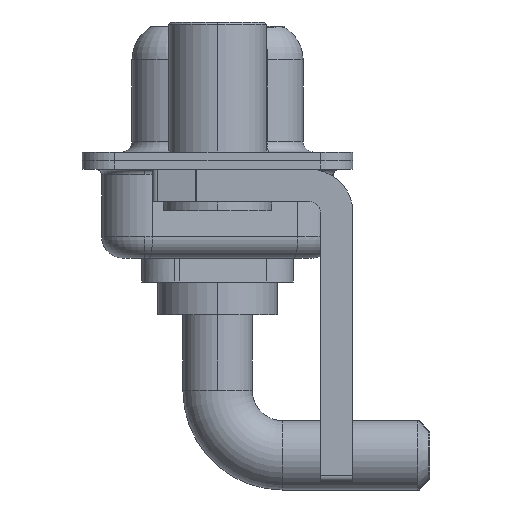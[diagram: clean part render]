
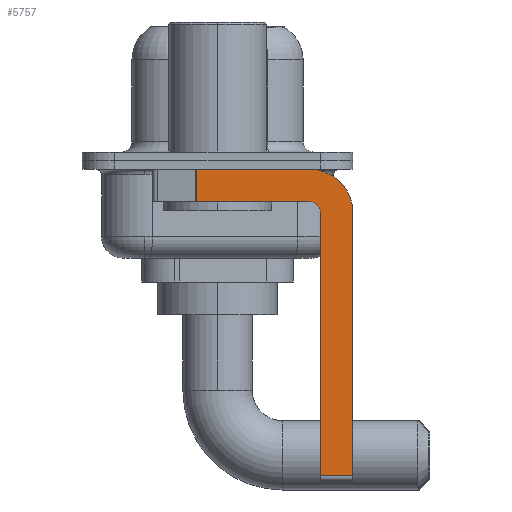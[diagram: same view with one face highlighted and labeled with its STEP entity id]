
A CAD part, left-side view. The second image highlights one B-rep face of the part: STEP entity #5757.
In plain terms, the highlighted planar face has unit normal (-1, 0, 0).
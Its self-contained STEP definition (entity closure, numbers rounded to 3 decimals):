
#242 = EDGE_CURVE ( 'NONE', #12646, #14776, #2877, .T. ) ;
#932 = CARTESIAN_POINT ( 'NONE',  ( -2.9, -6.25, -2.4 ) ) ;
#2519 = CARTESIAN_POINT ( 'NONE',  ( -2.9, -4.25, -1.9 ) ) ;
#2877 = LINE ( 'NONE', #10186, #12741 ) ;
#2991 = CIRCLE ( 'NONE', #9541, 2. ) ;
#3051 = VERTEX_POINT ( 'NONE', #7050 ) ;
#3181 = EDGE_LOOP ( 'NONE', ( #15367, #10333, #6201, #6462, #7003, #6808, #8947, #4265 ) ) ;
#3456 = CARTESIAN_POINT ( 'NONE',  ( -2.9, 0.978, -1.9 ) ) ;
#3582 = VERTEX_POINT ( 'NONE', #932 ) ;
#3919 = EDGE_CURVE ( 'NONE', #12646, #3051, #14127, .T. ) ;
#4265 = ORIENTED_EDGE ( 'NONE', *, *, #7021, .F. ) ;
#4307 = CARTESIAN_POINT ( 'NONE',  ( -2.9, -4.25, -14.55 ) ) ;
#4573 = VERTEX_POINT ( 'NONE', #7297 ) ;
#5104 = FACE_OUTER_BOUND ( 'NONE', #3181, .T. ) ;
#5132 = DIRECTION ( 'NONE',  ( 0., 0., -1. ) ) ;
#5217 = LINE ( 'NONE', #11481, #15758 ) ;
#5271 = LINE ( 'NONE', #9194, #6204 ) ;
#5757 = ADVANCED_FACE ( 'NONE', ( #5104 ), #8957, .F. ) ;
#5773 = AXIS2_PLACEMENT_3D ( 'NONE', #9042, #13033, #10471 ) ;
#6201 = ORIENTED_EDGE ( 'NONE', *, *, #6838, .F. ) ;
#6204 = VECTOR ( 'NONE', #9020, 1000. ) ;
#6462 = ORIENTED_EDGE ( 'NONE', *, *, #15039, .F. ) ;
#6474 = LINE ( 'NONE', #2519, #10650 ) ;
#6613 = DIRECTION ( 'NONE',  ( 0., -1., 0. ) ) ;
#6808 = ORIENTED_EDGE ( 'NONE', *, *, #3919, .T. ) ;
#6838 = EDGE_CURVE ( 'NONE', #8232, #13941, #6474, .T. ) ;
#7003 = ORIENTED_EDGE ( 'NONE', *, *, #242, .F. ) ;
#7021 = EDGE_CURVE ( 'NONE', #4573, #3582, #2991, .T. ) ;
#7050 = CARTESIAN_POINT ( 'NONE',  ( -2.9, -6.25, -14.55 ) ) ;
#7297 = CARTESIAN_POINT ( 'NONE',  ( -2.9, -4.25, -0.4 ) ) ;
#8232 = VERTEX_POINT ( 'NONE', #13463 ) ;
#8871 = EDGE_CURVE ( 'NONE', #13799, #13941, #13757, .T. ) ;
#8899 = CIRCLE ( 'NONE', #5773, 0.5 ) ;
#8947 = ORIENTED_EDGE ( 'NONE', *, *, #11909, .F. ) ;
#8957 = PLANE ( 'NONE',  #11171 ) ;
#9020 = DIRECTION ( 'NONE',  ( 0., -1., 0. ) ) ;
#9042 = CARTESIAN_POINT ( 'NONE',  ( -2.9, -4.25, -2.4 ) ) ;
#9194 = CARTESIAN_POINT ( 'NONE',  ( -2.9, 3., -0.4 ) ) ;
#9541 = AXIS2_PLACEMENT_3D ( 'NONE', #15632, #13074, #14486 ) ;
#10186 = CARTESIAN_POINT ( 'NONE',  ( -2.9, -4.75, -14.8 ) ) ;
#10281 = EDGE_CURVE ( 'NONE', #13799, #4573, #5271, .T. ) ;
#10333 = ORIENTED_EDGE ( 'NONE', *, *, #8871, .T. ) ;
#10471 = DIRECTION ( 'NONE',  ( 0., 0., 1. ) ) ;
#10650 = VECTOR ( 'NONE', #13903, 1000. ) ;
#10805 = CARTESIAN_POINT ( 'NONE',  ( -2.9, -4.75, -14.55 ) ) ;
#10818 = CARTESIAN_POINT ( 'NONE',  ( -2.9, -4.75, -2.4 ) ) ;
#11171 = AXIS2_PLACEMENT_3D ( 'NONE', #13857, #14026, #15338 ) ;
#11436 = DIRECTION ( 'NONE',  ( 0., 0., 1. ) ) ;
#11481 = CARTESIAN_POINT ( 'NONE',  ( -2.9, -6.25, -2.4 ) ) ;
#11909 = EDGE_CURVE ( 'NONE', #3582, #3051, #5217, .T. ) ;
#12351 = DIRECTION ( 'NONE',  ( 0., 0., -1. ) ) ;
#12646 = VERTEX_POINT ( 'NONE', #10805 ) ;
#12741 = VECTOR ( 'NONE', #11436, 1000. ) ;
#12960 = CARTESIAN_POINT ( 'NONE',  ( -2.9, 0.978, -1.9 ) ) ;
#13033 = DIRECTION ( 'NONE',  ( -1., 0., 0. ) ) ;
#13074 = DIRECTION ( 'NONE',  ( 1., 0., 0. ) ) ;
#13463 = CARTESIAN_POINT ( 'NONE',  ( -2.9, -4.25, -1.9 ) ) ;
#13757 = LINE ( 'NONE', #3456, #14361 ) ;
#13799 = VERTEX_POINT ( 'NONE', #14860 ) ;
#13857 = CARTESIAN_POINT ( 'NONE',  ( -2.9, -4.25, -2.4 ) ) ;
#13903 = DIRECTION ( 'NONE',  ( 0., 1., 0. ) ) ;
#13941 = VERTEX_POINT ( 'NONE', #12960 ) ;
#14026 = DIRECTION ( 'NONE',  ( 1., 0., 0. ) ) ;
#14127 = LINE ( 'NONE', #4307, #15802 ) ;
#14361 = VECTOR ( 'NONE', #12351, 1000. ) ;
#14486 = DIRECTION ( 'NONE',  ( 0., 0., -1. ) ) ;
#14776 = VERTEX_POINT ( 'NONE', #10818 ) ;
#14860 = CARTESIAN_POINT ( 'NONE',  ( -2.9, 0.978, -0.4 ) ) ;
#15039 = EDGE_CURVE ( 'NONE', #14776, #8232, #8899, .T. ) ;
#15338 = DIRECTION ( 'NONE',  ( 0., 0., -1. ) ) ;
#15367 = ORIENTED_EDGE ( 'NONE', *, *, #10281, .F. ) ;
#15632 = CARTESIAN_POINT ( 'NONE',  ( -2.9, -4.25, -2.4 ) ) ;
#15758 = VECTOR ( 'NONE', #5132, 1000. ) ;
#15802 = VECTOR ( 'NONE', #6613, 1000. ) ;
